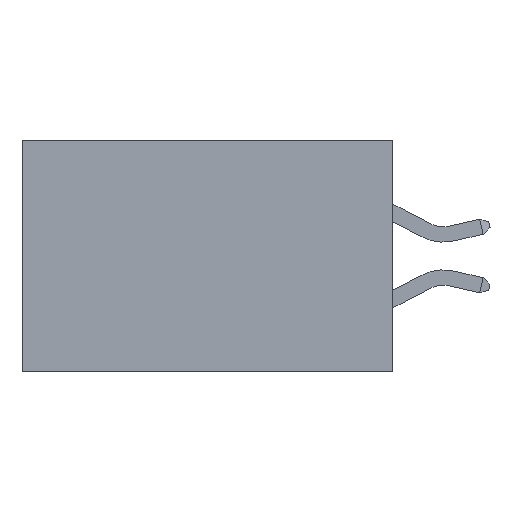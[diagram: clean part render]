
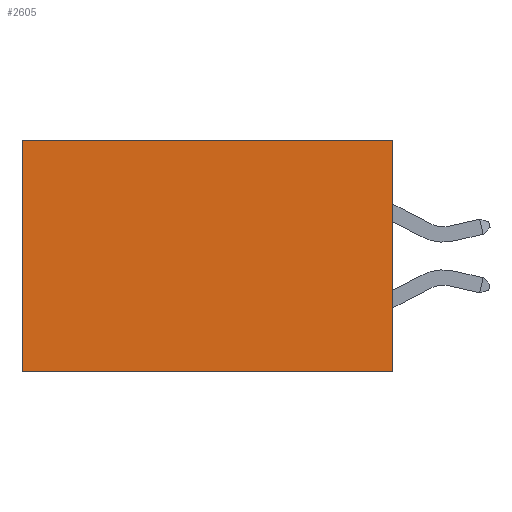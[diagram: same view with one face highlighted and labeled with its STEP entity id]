
A CAD part, left-side view. The second image highlights one B-rep face of the part: STEP entity #2605.
In plain terms, the highlighted planar face has unit normal (-1, 0, 0).
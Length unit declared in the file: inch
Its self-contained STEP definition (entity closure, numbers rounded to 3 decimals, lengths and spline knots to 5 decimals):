
#228 = VERTEX_POINT ( 'NONE', #7831 ) ;
#998 = DIRECTION ( 'NONE',  ( 0., 0., -1. ) ) ;
#1385 = VERTEX_POINT ( 'NONE', #9169 ) ;
#1714 = EDGE_CURVE ( 'NONE', #1385, #15278, #12278, .T. ) ;
#1843 = VECTOR ( 'NONE', #14206, 39.37008 ) ;
#2543 = LINE ( 'NONE', #5672, #10269 ) ;
#2605 = ADVANCED_FACE ( 'NONE', ( #15610 ), #17834, .F. ) ;
#3579 = EDGE_CURVE ( 'NONE', #6368, #15278, #2543, .T. ) ;
#3588 = CARTESIAN_POINT ( 'NONE',  ( 0.2875, 0., -0.375 ) ) ;
#4622 = ORIENTED_EDGE ( 'NONE', *, *, #3579, .F. ) ;
#4828 = AXIS2_PLACEMENT_3D ( 'NONE', #3588, #9167, #998 ) ;
#5609 = EDGE_CURVE ( 'NONE', #228, #1385, #10418, .T. ) ;
#5672 = CARTESIAN_POINT ( 'NONE',  ( 0.2875, 0., -0.375 ) ) ;
#6356 = EDGE_LOOP ( 'NONE', ( #7914, #4622, #15732, #13076 ) ) ;
#6368 = VERTEX_POINT ( 'NONE', #8592 ) ;
#7073 = CARTESIAN_POINT ( 'NONE',  ( 0.2875, 0.6, -0.375 ) ) ;
#7618 = CARTESIAN_POINT ( 'NONE',  ( 0.2875, 0., 0. ) ) ;
#7831 = CARTESIAN_POINT ( 'NONE',  ( 0.2875, 0., 0. ) ) ;
#7914 = ORIENTED_EDGE ( 'NONE', *, *, #1714, .T. ) ;
#8592 = CARTESIAN_POINT ( 'NONE',  ( 0.2875, 0., -0.375 ) ) ;
#9031 = DIRECTION ( 'NONE',  ( 0., 0., -1. ) ) ;
#9167 = DIRECTION ( 'NONE',  ( 1., 0., 0. ) ) ;
#9169 = CARTESIAN_POINT ( 'NONE',  ( 0.2875, 0.6, 0. ) ) ;
#9268 = DIRECTION ( 'NONE',  ( 0., 1., 0. ) ) ;
#10269 = VECTOR ( 'NONE', #15771, 39.37008 ) ;
#10418 = LINE ( 'NONE', #7618, #15815 ) ;
#11880 = CARTESIAN_POINT ( 'NONE',  ( 0.2875, 0., -0.375 ) ) ;
#12278 = LINE ( 'NONE', #7073, #1843 ) ;
#13076 = ORIENTED_EDGE ( 'NONE', *, *, #5609, .T. ) ;
#13956 = EDGE_CURVE ( 'NONE', #228, #6368, #18371, .T. ) ;
#14206 = DIRECTION ( 'NONE',  ( 0., 0., -1. ) ) ;
#15278 = VERTEX_POINT ( 'NONE', #16663 ) ;
#15610 = FACE_OUTER_BOUND ( 'NONE', #6356, .T. ) ;
#15732 = ORIENTED_EDGE ( 'NONE', *, *, #13956, .F. ) ;
#15771 = DIRECTION ( 'NONE',  ( 0., 1., 0. ) ) ;
#15815 = VECTOR ( 'NONE', #9268, 39.37008 ) ;
#16663 = CARTESIAN_POINT ( 'NONE',  ( 0.2875, 0.6, -0.375 ) ) ;
#17487 = VECTOR ( 'NONE', #9031, 39.37008 ) ;
#17834 = PLANE ( 'NONE',  #4828 ) ;
#18371 = LINE ( 'NONE', #11880, #17487 ) ;
